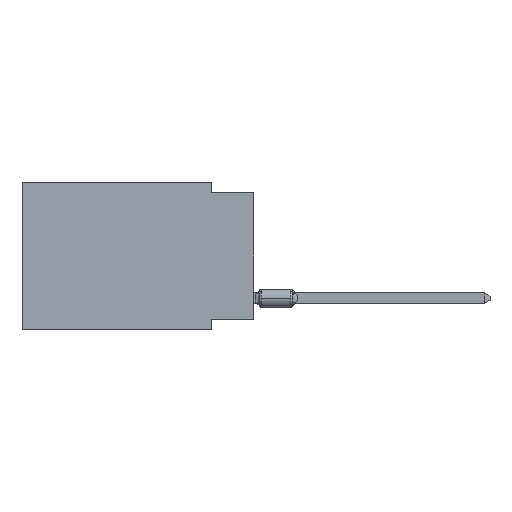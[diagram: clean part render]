
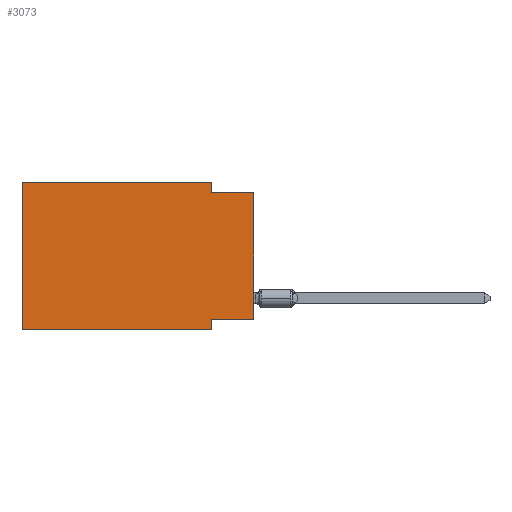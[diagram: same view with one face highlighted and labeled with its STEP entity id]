
A CAD part, left-side view. The second image highlights one B-rep face of the part: STEP entity #3073.
In plain terms, the highlighted planar face has unit normal (-1, 0, 0).
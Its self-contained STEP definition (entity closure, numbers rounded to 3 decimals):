
#170 = EDGE_CURVE ( 'NONE', #16497, #24786, #16694, .T. ) ;
#429 = LINE ( 'NONE', #7754, #7172 ) ;
#985 = CARTESIAN_POINT ( 'NONE',  ( 0., 2.54, 0. ) ) ;
#1669 = LINE ( 'NONE', #31121, #27739 ) ;
#2019 = CARTESIAN_POINT ( 'NONE',  ( 0., 13.97, 0. ) ) ;
#2196 = FACE_OUTER_BOUND ( 'NONE', #3169, .T. ) ;
#2481 = VERTEX_POINT ( 'NONE', #31186 ) ;
#3073 = ADVANCED_FACE ( 'NONE', ( #2196 ), #26552, .F. ) ;
#3169 = EDGE_LOOP ( 'NONE', ( #18367, #14402, #22125, #13385, #9036, #6176, #20403, #5468 ) ) ;
#3510 = VECTOR ( 'NONE', #30171, 1000. ) ;
#4148 = VERTEX_POINT ( 'NONE', #985 ) ;
#4736 = VECTOR ( 'NONE', #8178, 1000. ) ;
#5153 = CARTESIAN_POINT ( 'NONE',  ( 0., 0., 0. ) ) ;
#5468 = ORIENTED_EDGE ( 'NONE', *, *, #170, .F. ) ;
#6176 = ORIENTED_EDGE ( 'NONE', *, *, #15337, .T. ) ;
#6833 = CARTESIAN_POINT ( 'NONE',  ( 0., 0., -8.255 ) ) ;
#7172 = VECTOR ( 'NONE', #9666, 1000. ) ;
#7745 = LINE ( 'NONE', #10598, #3510 ) ;
#7754 = CARTESIAN_POINT ( 'NONE',  ( 0., 13.97, -8.89 ) ) ;
#8178 = DIRECTION ( 'NONE',  ( 0., 0., -1. ) ) ;
#8790 = LINE ( 'NONE', #30445, #4736 ) ;
#9036 = ORIENTED_EDGE ( 'NONE', *, *, #23700, .F. ) ;
#9666 = DIRECTION ( 'NONE',  ( 0., -1., 0. ) ) ;
#9673 = CARTESIAN_POINT ( 'NONE',  ( 0., 0., -8.255 ) ) ;
#9839 = DIRECTION ( 'NONE',  ( 0., 0., -1. ) ) ;
#10230 = VECTOR ( 'NONE', #31022, 1000. ) ;
#10598 = CARTESIAN_POINT ( 'NONE',  ( 0., 0., -0.635 ) ) ;
#11252 = EDGE_CURVE ( 'NONE', #16497, #2481, #17251, .T. ) ;
#12791 = CARTESIAN_POINT ( 'NONE',  ( 0., 2.54, -0.635 ) ) ;
#12861 = EDGE_CURVE ( 'NONE', #4148, #20992, #1669, .T. ) ;
#13385 = ORIENTED_EDGE ( 'NONE', *, *, #30929, .F. ) ;
#14175 = VECTOR ( 'NONE', #20379, 1000. ) ;
#14402 = ORIENTED_EDGE ( 'NONE', *, *, #31268, .F. ) ;
#14861 = DIRECTION ( 'NONE',  ( 0., 0., 1. ) ) ;
#15337 = EDGE_CURVE ( 'NONE', #21426, #22160, #429, .T. ) ;
#15910 = LINE ( 'NONE', #2019, #14175 ) ;
#15962 = VERTEX_POINT ( 'NONE', #29985 ) ;
#16497 = VERTEX_POINT ( 'NONE', #9673 ) ;
#16694 = LINE ( 'NONE', #6833, #10230 ) ;
#17251 = LINE ( 'NONE', #5153, #26600 ) ;
#17328 = CARTESIAN_POINT ( 'NONE',  ( 0., 13.97, 0. ) ) ;
#18367 = ORIENTED_EDGE ( 'NONE', *, *, #11252, .T. ) ;
#18713 = DIRECTION ( 'NONE',  ( 0., 0., -1. ) ) ;
#19419 = AXIS2_PLACEMENT_3D ( 'NONE', #24175, #24331, #9839 ) ;
#20379 = DIRECTION ( 'NONE',  ( 0., -1., 0. ) ) ;
#20403 = ORIENTED_EDGE ( 'NONE', *, *, #21220, .F. ) ;
#20853 = CARTESIAN_POINT ( 'NONE',  ( 0., 2.54, -8.89 ) ) ;
#20992 = VERTEX_POINT ( 'NONE', #12791 ) ;
#21220 = EDGE_CURVE ( 'NONE', #24786, #22160, #8790, .T. ) ;
#21426 = VERTEX_POINT ( 'NONE', #21994 ) ;
#21994 = CARTESIAN_POINT ( 'NONE',  ( 0., 13.97, -8.89 ) ) ;
#22125 = ORIENTED_EDGE ( 'NONE', *, *, #12861, .F. ) ;
#22160 = VERTEX_POINT ( 'NONE', #20853 ) ;
#23700 = EDGE_CURVE ( 'NONE', #21426, #15962, #29433, .T. ) ;
#23772 = CARTESIAN_POINT ( 'NONE',  ( 0., 2.54, -8.255 ) ) ;
#24175 = CARTESIAN_POINT ( 'NONE',  ( 0., 13.97, 0. ) ) ;
#24331 = DIRECTION ( 'NONE',  ( 1., 0., 0. ) ) ;
#24786 = VERTEX_POINT ( 'NONE', #23772 ) ;
#26552 = PLANE ( 'NONE',  #19419 ) ;
#26600 = VECTOR ( 'NONE', #14861, 1000. ) ;
#27048 = DIRECTION ( 'NONE',  ( 0., 0., 1. ) ) ;
#27739 = VECTOR ( 'NONE', #18713, 1000. ) ;
#29433 = LINE ( 'NONE', #17328, #30184 ) ;
#29985 = CARTESIAN_POINT ( 'NONE',  ( 0., 13.97, 0. ) ) ;
#30171 = DIRECTION ( 'NONE',  ( 0., -1., 0. ) ) ;
#30184 = VECTOR ( 'NONE', #27048, 1000. ) ;
#30445 = CARTESIAN_POINT ( 'NONE',  ( 0., 2.54, -8.89 ) ) ;
#30929 = EDGE_CURVE ( 'NONE', #15962, #4148, #15910, .T. ) ;
#31022 = DIRECTION ( 'NONE',  ( 0., 1., 0. ) ) ;
#31121 = CARTESIAN_POINT ( 'NONE',  ( 0., 2.54, 0. ) ) ;
#31186 = CARTESIAN_POINT ( 'NONE',  ( 0., 0., -0.635 ) ) ;
#31268 = EDGE_CURVE ( 'NONE', #20992, #2481, #7745, .T. ) ;
